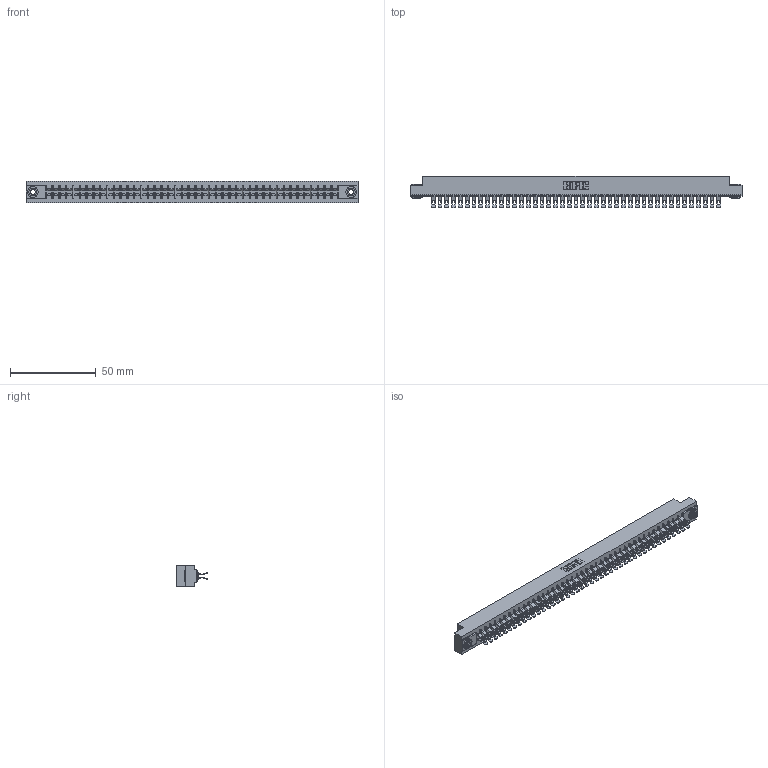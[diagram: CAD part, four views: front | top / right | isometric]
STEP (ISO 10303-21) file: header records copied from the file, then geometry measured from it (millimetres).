
FILE_DESCRIPTION (( 'STEP AP203' ), '1' );
FILE_NAME ('305-086-555-203.STEP', '2019-09-10T12:58:51', ( '' ), ( '' ), 'SwSTEP 2.0', 'SolidWorks 2016', '' );
FILE_SCHEMA (( 'CONFIG_CONTROL_DESIGN' ));
Length unit declared in the file: inch
Products named in the file (4): 305-290-001_555; 345-250-002_345-250-002-102; 305 Part_.156 Dia; 305-086-555-203
Assembly tree (89 placements, depth 2):
  305-086-555-203
    305 Part_.156 Dia
    305-290-001_555  x86
    345-250-002_345-250-002-102  x2
Bounding box: 193.4 x 18.41 x 12.7 mm (x, y, z)
Volume: 20430.1 mm3; surface area: 27898.9 mm2
Topology: 89 solids, 89 shells, 5844 faces, 17413 edges, 11374 vertices
Faces by surface type: plane 2844, cylinder 2820, sphere 172, cone 8
Entity records: 48125 total; most frequent: CARTESIAN_POINT 7962, ORIENTED_EDGE 7886, DIRECTION 7711, EDGE_CURVE 3943, VECTOR 3161, LINE 3161, VERTEX_POINT 2510, AXIS2_PLACEMENT_3D 2275
